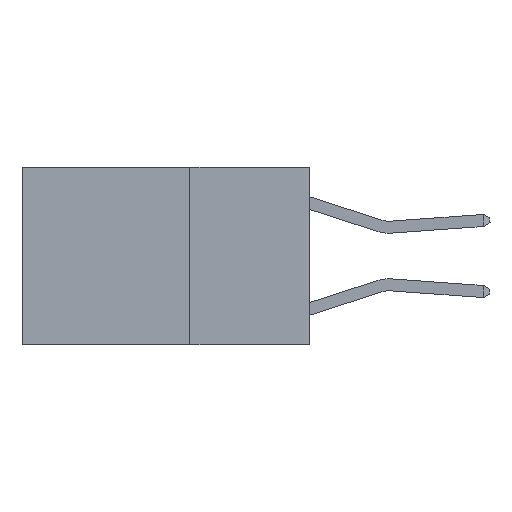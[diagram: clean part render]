
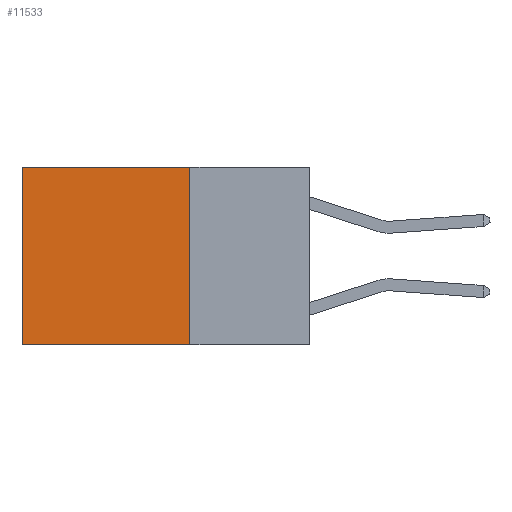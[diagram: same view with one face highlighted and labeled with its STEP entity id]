
A CAD part, left-side view. The second image highlights one B-rep face of the part: STEP entity #11533.
In plain terms, the highlighted planar face has unit normal (-1, 0, 0).
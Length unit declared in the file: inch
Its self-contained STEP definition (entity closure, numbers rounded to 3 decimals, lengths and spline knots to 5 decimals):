
#687 = VERTEX_POINT ( 'NONE', #8033 ) ;
#3746 = VERTEX_POINT ( 'NONE', #25598 ) ;
#3898 = ORIENTED_EDGE ( 'NONE', *, *, #20741, .T. ) ;
#4218 = FACE_OUTER_BOUND ( 'NONE', #9843, .T. ) ;
#4557 = EDGE_CURVE ( 'NONE', #3746, #24324, #14754, .T. ) ;
#6990 = DIRECTION ( 'NONE',  ( 0., 0., -1. ) ) ;
#7387 = VERTEX_POINT ( 'NONE', #19826 ) ;
#8033 = CARTESIAN_POINT ( 'NONE',  ( 0.2625, 0.25, -0.37 ) ) ;
#8374 = VECTOR ( 'NONE', #15256, 39.37008 ) ;
#8375 = LINE ( 'NONE', #10549, #22318 ) ;
#9080 = LINE ( 'NONE', #18619, #8374 ) ;
#9431 = LINE ( 'NONE', #17138, #21985 ) ;
#9843 = EDGE_LOOP ( 'NONE', ( #22014, #15201, #13396, #3898 ) ) ;
#9910 = EDGE_CURVE ( 'NONE', #7387, #687, #8375, .T. ) ;
#10549 = CARTESIAN_POINT ( 'NONE',  ( 0.2625, 0.25, 0. ) ) ;
#11533 = ADVANCED_FACE ( 'NONE', ( #4218 ), #13698, .F. ) ;
#13396 = ORIENTED_EDGE ( 'NONE', *, *, #9910, .F. ) ;
#13464 = CARTESIAN_POINT ( 'NONE',  ( 0.2625, 0.6, -0.37 ) ) ;
#13531 = AXIS2_PLACEMENT_3D ( 'NONE', #13938, #17666, #19499 ) ;
#13698 = PLANE ( 'NONE',  #13531 ) ;
#13938 = CARTESIAN_POINT ( 'NONE',  ( 0.2625, 0.25, 0. ) ) ;
#14754 = LINE ( 'NONE', #22629, #21816 ) ;
#15201 = ORIENTED_EDGE ( 'NONE', *, *, #20036, .F. ) ;
#15256 = DIRECTION ( 'NONE',  ( 0., 1., 0. ) ) ;
#17138 = CARTESIAN_POINT ( 'NONE',  ( 0.2625, 0.25, 0. ) ) ;
#17666 = DIRECTION ( 'NONE',  ( 1., 0., 0. ) ) ;
#18415 = DIRECTION ( 'NONE',  ( 0., 0., -1. ) ) ;
#18619 = CARTESIAN_POINT ( 'NONE',  ( 0.2625, 0.25, -0.37 ) ) ;
#19499 = DIRECTION ( 'NONE',  ( 0., 0., -1. ) ) ;
#19826 = CARTESIAN_POINT ( 'NONE',  ( 0.2625, 0.25, 0. ) ) ;
#20036 = EDGE_CURVE ( 'NONE', #687, #24324, #9080, .T. ) ;
#20741 = EDGE_CURVE ( 'NONE', #7387, #3746, #9431, .T. ) ;
#21816 = VECTOR ( 'NONE', #6990, 39.37008 ) ;
#21985 = VECTOR ( 'NONE', #25073, 39.37008 ) ;
#22014 = ORIENTED_EDGE ( 'NONE', *, *, #4557, .T. ) ;
#22318 = VECTOR ( 'NONE', #18415, 39.37008 ) ;
#22629 = CARTESIAN_POINT ( 'NONE',  ( 0.2625, 0.6, 0. ) ) ;
#24324 = VERTEX_POINT ( 'NONE', #13464 ) ;
#25073 = DIRECTION ( 'NONE',  ( 0., 1., 0. ) ) ;
#25598 = CARTESIAN_POINT ( 'NONE',  ( 0.2625, 0.6, 0. ) ) ;
